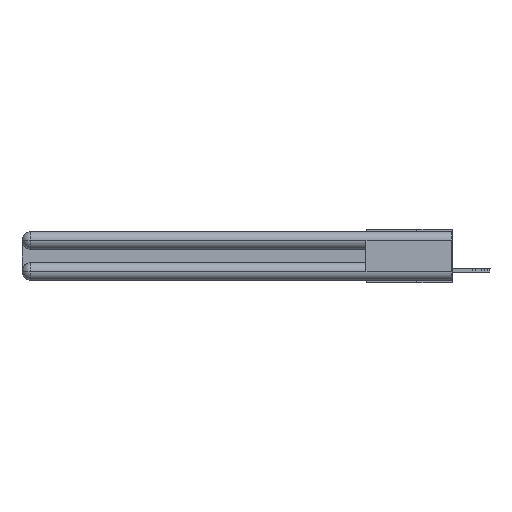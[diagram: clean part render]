
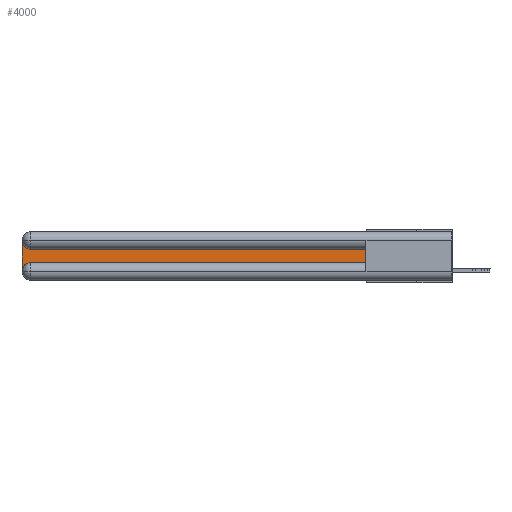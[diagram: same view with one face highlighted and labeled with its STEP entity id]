
A CAD part, left-side view. The second image highlights one B-rep face of the part: STEP entity #4000.
In plain terms, the highlighted planar face has unit normal (-1, 0, 0).
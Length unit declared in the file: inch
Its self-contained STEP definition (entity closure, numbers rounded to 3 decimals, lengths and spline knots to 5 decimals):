
#94 = VERTEX_POINT ( 'NONE', #7272 ) ;
#339 = CIRCLE ( 'NONE', #5222, 0.06 ) ;
#623 = CARTESIAN_POINT ( 'NONE',  ( 0.075, 2.94, -0.2775 ) ) ;
#894 = DIRECTION ( 'NONE',  ( 0., 0., 1. ) ) ;
#1894 = DIRECTION ( 'NONE',  ( 0., 0., -1. ) ) ;
#2278 = VERTEX_POINT ( 'NONE', #9129 ) ;
#2324 = EDGE_CURVE ( 'NONE', #7177, #11783, #8520, .T. ) ;
#2580 = PLANE ( 'NONE',  #11341 ) ;
#2883 = EDGE_LOOP ( 'NONE', ( #15079, #26232, #4443, #4002, #5924, #15603 ) ) ;
#3384 = LINE ( 'NONE', #25222, #26540 ) ;
#4000 = ADVANCED_FACE ( 'NONE', ( #8458 ), #2580, .F. ) ;
#4002 = ORIENTED_EDGE ( 'NONE', *, *, #4422, .T. ) ;
#4422 = EDGE_CURVE ( 'NONE', #5255, #94, #339, .T. ) ;
#4436 = LINE ( 'NONE', #9545, #24045 ) ;
#4443 = ORIENTED_EDGE ( 'NONE', *, *, #25808, .T. ) ;
#5222 = AXIS2_PLACEMENT_3D ( 'NONE', #623, #25692, #8960 ) ;
#5255 = VERTEX_POINT ( 'NONE', #9094 ) ;
#5924 = ORIENTED_EDGE ( 'NONE', *, *, #23602, .T. ) ;
#6747 = CARTESIAN_POINT ( 'NONE',  ( 0.075, 3., -0.1225 ) ) ;
#7177 = VERTEX_POINT ( 'NONE', #7779 ) ;
#7272 = CARTESIAN_POINT ( 'NONE',  ( 0.075, 2.94, -0.2175 ) ) ;
#7397 = CARTESIAN_POINT ( 'NONE',  ( 0.075, 0.6, -0.2175 ) ) ;
#7779 = CARTESIAN_POINT ( 'NONE',  ( 0.075, 0.6, -0.2175 ) ) ;
#7845 = DIRECTION ( 'NONE',  ( 1., 0., 0. ) ) ;
#8326 = CARTESIAN_POINT ( 'NONE',  ( 0.075, 3., -0.2175 ) ) ;
#8458 = FACE_OUTER_BOUND ( 'NONE', #2883, .T. ) ;
#8520 = LINE ( 'NONE', #7397, #17384 ) ;
#8960 = DIRECTION ( 'NONE',  ( 0., 0., -1. ) ) ;
#9094 = CARTESIAN_POINT ( 'NONE',  ( 0.075, 3., -0.2775 ) ) ;
#9129 = CARTESIAN_POINT ( 'NONE',  ( 0.075, 3., -0.0625 ) ) ;
#9545 = CARTESIAN_POINT ( 'NONE',  ( 0.075, 0.6, -0.2175 ) ) ;
#11122 = VERTEX_POINT ( 'NONE', #18192 ) ;
#11341 = AXIS2_PLACEMENT_3D ( 'NONE', #6747, #7845, #24498 ) ;
#11783 = VERTEX_POINT ( 'NONE', #25625 ) ;
#12158 = EDGE_CURVE ( 'NONE', #11783, #11122, #3384, .T. ) ;
#14754 = LINE ( 'NONE', #8326, #16074 ) ;
#14917 = DIRECTION ( 'NONE',  ( 1., 0., 0. ) ) ;
#15079 = ORIENTED_EDGE ( 'NONE', *, *, #12158, .T. ) ;
#15587 = AXIS2_PLACEMENT_3D ( 'NONE', #23414, #14917, #17027 ) ;
#15603 = ORIENTED_EDGE ( 'NONE', *, *, #2324, .T. ) ;
#16074 = VECTOR ( 'NONE', #1894, 39.37008 ) ;
#17027 = DIRECTION ( 'NONE',  ( 0., 0., -1. ) ) ;
#17384 = VECTOR ( 'NONE', #894, 39.37008 ) ;
#18192 = CARTESIAN_POINT ( 'NONE',  ( 0.075, 2.94, -0.1225 ) ) ;
#18903 = EDGE_CURVE ( 'NONE', #11122, #2278, #21819, .T. ) ;
#19016 = DIRECTION ( 'NONE',  ( 0., 1., 0. ) ) ;
#21819 = CIRCLE ( 'NONE', #15587, 0.06 ) ;
#23414 = CARTESIAN_POINT ( 'NONE',  ( 0.075, 2.94, -0.0625 ) ) ;
#23602 = EDGE_CURVE ( 'NONE', #94, #7177, #4436, .T. ) ;
#24045 = VECTOR ( 'NONE', #26275, 39.37008 ) ;
#24498 = DIRECTION ( 'NONE',  ( 0., 0., -1. ) ) ;
#25222 = CARTESIAN_POINT ( 'NONE',  ( 0.075, 0.6, -0.1225 ) ) ;
#25625 = CARTESIAN_POINT ( 'NONE',  ( 0.075, 0.6, -0.1225 ) ) ;
#25692 = DIRECTION ( 'NONE',  ( 1., 0., 0. ) ) ;
#25808 = EDGE_CURVE ( 'NONE', #2278, #5255, #14754, .T. ) ;
#26232 = ORIENTED_EDGE ( 'NONE', *, *, #18903, .T. ) ;
#26275 = DIRECTION ( 'NONE',  ( 0., -1., 0. ) ) ;
#26540 = VECTOR ( 'NONE', #19016, 39.37008 ) ;
